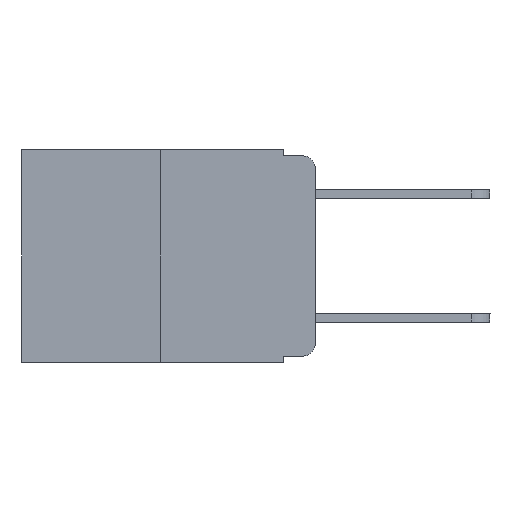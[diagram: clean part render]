
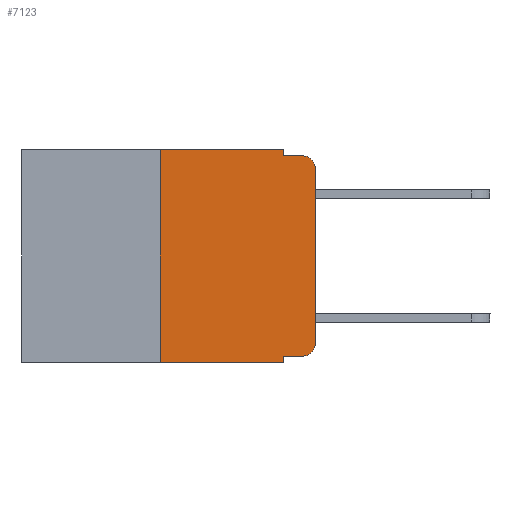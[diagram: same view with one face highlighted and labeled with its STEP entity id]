
A CAD part, left-side view. The second image highlights one B-rep face of the part: STEP entity #7123.
In plain terms, the highlighted planar face has unit normal (-1, 0, 0).
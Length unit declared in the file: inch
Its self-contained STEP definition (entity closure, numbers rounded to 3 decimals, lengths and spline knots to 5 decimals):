
#103 = CARTESIAN_POINT ( 'NONE',  ( 0., 0.051, -0.01 ) ) ;
#338 = EDGE_CURVE ( 'NONE', #5056, #12515, #9821, .T. ) ;
#601 = EDGE_CURVE ( 'NONE', #4877, #5056, #4634, .T. ) ;
#730 = AXIS2_PLACEMENT_3D ( 'NONE', #5158, #6620, #910 ) ;
#858 = VECTOR ( 'NONE', #16712, 39.37008 ) ;
#910 = DIRECTION ( 'NONE',  ( 0., 0., -1. ) ) ;
#985 = CARTESIAN_POINT ( 'NONE',  ( 0., 0., 0. ) ) ;
#1164 = CARTESIAN_POINT ( 'NONE',  ( 0., 0.02, -0.333 ) ) ;
#1464 = ORIENTED_EDGE ( 'NONE', *, *, #12549, .T. ) ;
#2053 = CARTESIAN_POINT ( 'NONE',  ( 0., 0.051, -0.333 ) ) ;
#2313 = VERTEX_POINT ( 'NONE', #17338 ) ;
#2677 = CARTESIAN_POINT ( 'NONE',  ( 0., 0.02, -0.03 ) ) ;
#2783 = ORIENTED_EDGE ( 'NONE', *, *, #601, .T. ) ;
#2839 = ORIENTED_EDGE ( 'NONE', *, *, #5489, .F. ) ;
#2939 = ORIENTED_EDGE ( 'NONE', *, *, #3063, .F. ) ;
#3063 = EDGE_CURVE ( 'NONE', #14599, #2313, #13198, .T. ) ;
#3427 = DIRECTION ( 'NONE',  ( 0., -1., 0. ) ) ;
#4075 = FACE_OUTER_BOUND ( 'NONE', #4089, .T. ) ;
#4089 = EDGE_LOOP ( 'NONE', ( #8130, #1464, #14038, #5723, #2939, #2839, #5693, #18598, #7907, #2783 ) ) ;
#4294 = VECTOR ( 'NONE', #9992, 39.37008 ) ;
#4368 = CARTESIAN_POINT ( 'NONE',  ( 0., 0.25, -0.343 ) ) ;
#4545 = LINE ( 'NONE', #12502, #15597 ) ;
#4634 = CIRCLE ( 'NONE', #11549, 0.02 ) ;
#4877 = VERTEX_POINT ( 'NONE', #1164 ) ;
#5056 = VERTEX_POINT ( 'NONE', #16783 ) ;
#5158 = CARTESIAN_POINT ( 'NONE',  ( 0., 0.473, 0. ) ) ;
#5489 = EDGE_CURVE ( 'NONE', #18479, #14599, #15844, .T. ) ;
#5693 = ORIENTED_EDGE ( 'NONE', *, *, #10794, .T. ) ;
#5723 = ORIENTED_EDGE ( 'NONE', *, *, #18448, .F. ) ;
#5733 = CARTESIAN_POINT ( 'NONE',  ( 0., 0.051, 0. ) ) ;
#6059 = VECTOR ( 'NONE', #7206, 39.37008 ) ;
#6181 = AXIS2_PLACEMENT_3D ( 'NONE', #2677, #12671, #7006 ) ;
#6620 = DIRECTION ( 'NONE',  ( 1., 0., 0. ) ) ;
#6659 = CARTESIAN_POINT ( 'NONE',  ( 0., 0.473, 0. ) ) ;
#6785 = DIRECTION ( 'NONE',  ( -1., 0., 0. ) ) ;
#7006 = DIRECTION ( 'NONE',  ( 0., 0., -1. ) ) ;
#7123 = ADVANCED_FACE ( 'NONE', ( #4075 ), #15305, .F. ) ;
#7206 = DIRECTION ( 'NONE',  ( 0., 0., -1. ) ) ;
#7907 = ORIENTED_EDGE ( 'NONE', *, *, #10437, .T. ) ;
#7943 = VECTOR ( 'NONE', #9823, 39.37008 ) ;
#8130 = ORIENTED_EDGE ( 'NONE', *, *, #338, .T. ) ;
#8145 = VERTEX_POINT ( 'NONE', #13775 ) ;
#8562 = VECTOR ( 'NONE', #13264, 39.37008 ) ;
#8959 = VERTEX_POINT ( 'NONE', #9452 ) ;
#9452 = CARTESIAN_POINT ( 'NONE',  ( 0., 0.02, -0.01 ) ) ;
#9455 = LINE ( 'NONE', #2053, #16924 ) ;
#9636 = DIRECTION ( 'NONE',  ( 0., 0., -1. ) ) ;
#9742 = VERTEX_POINT ( 'NONE', #14887 ) ;
#9821 = LINE ( 'NONE', #985, #17036 ) ;
#9823 = DIRECTION ( 'NONE',  ( 0., 0., 1. ) ) ;
#9930 = CARTESIAN_POINT ( 'NONE',  ( 0., 0.473, -0.343 ) ) ;
#9992 = DIRECTION ( 'NONE',  ( 0., -1., 0. ) ) ;
#10437 = EDGE_CURVE ( 'NONE', #8145, #4877, #9455, .T. ) ;
#10467 = CARTESIAN_POINT ( 'NONE',  ( 0., 0.051, -0.01 ) ) ;
#10681 = EDGE_CURVE ( 'NONE', #8145, #9742, #4545, .T. ) ;
#10794 = EDGE_CURVE ( 'NONE', #18479, #9742, #13992, .T. ) ;
#11438 = CARTESIAN_POINT ( 'NONE',  ( 0., 0.25, 0. ) ) ;
#11549 = AXIS2_PLACEMENT_3D ( 'NONE', #18409, #6785, #9636 ) ;
#11651 = CIRCLE ( 'NONE', #6181, 0.02 ) ;
#12502 = CARTESIAN_POINT ( 'NONE',  ( 0., 0.051, 0. ) ) ;
#12515 = VERTEX_POINT ( 'NONE', #15614 ) ;
#12549 = EDGE_CURVE ( 'NONE', #12515, #8959, #11651, .T. ) ;
#12671 = DIRECTION ( 'NONE',  ( -1., 0., 0. ) ) ;
#13198 = LINE ( 'NONE', #6659, #858 ) ;
#13264 = DIRECTION ( 'NONE',  ( 0., -1., 0. ) ) ;
#13775 = CARTESIAN_POINT ( 'NONE',  ( 0., 0.051, -0.333 ) ) ;
#13983 = DIRECTION ( 'NONE',  ( 0., 0., -1. ) ) ;
#13992 = LINE ( 'NONE', #9930, #8562 ) ;
#14038 = ORIENTED_EDGE ( 'NONE', *, *, #18415, .F. ) ;
#14204 = LINE ( 'NONE', #103, #4294 ) ;
#14599 = VERTEX_POINT ( 'NONE', #18043 ) ;
#14887 = CARTESIAN_POINT ( 'NONE',  ( 0., 0.051, -0.343 ) ) ;
#15305 = PLANE ( 'NONE',  #730 ) ;
#15597 = VECTOR ( 'NONE', #13983, 39.37008 ) ;
#15614 = CARTESIAN_POINT ( 'NONE',  ( 0., 0., -0.03 ) ) ;
#15844 = LINE ( 'NONE', #11438, #7943 ) ;
#16355 = VERTEX_POINT ( 'NONE', #10467 ) ;
#16422 = LINE ( 'NONE', #5733, #6059 ) ;
#16712 = DIRECTION ( 'NONE',  ( 0., -1., 0. ) ) ;
#16783 = CARTESIAN_POINT ( 'NONE',  ( 0., 0., -0.313 ) ) ;
#16924 = VECTOR ( 'NONE', #3427, 39.37008 ) ;
#16987 = DIRECTION ( 'NONE',  ( 0., 0., 1. ) ) ;
#17036 = VECTOR ( 'NONE', #16987, 39.37008 ) ;
#17338 = CARTESIAN_POINT ( 'NONE',  ( 0., 0.051, 0. ) ) ;
#18043 = CARTESIAN_POINT ( 'NONE',  ( 0., 0.25, 0. ) ) ;
#18409 = CARTESIAN_POINT ( 'NONE',  ( 0., 0.02, -0.313 ) ) ;
#18415 = EDGE_CURVE ( 'NONE', #16355, #8959, #14204, .T. ) ;
#18448 = EDGE_CURVE ( 'NONE', #2313, #16355, #16422, .T. ) ;
#18479 = VERTEX_POINT ( 'NONE', #4368 ) ;
#18598 = ORIENTED_EDGE ( 'NONE', *, *, #10681, .F. ) ;
